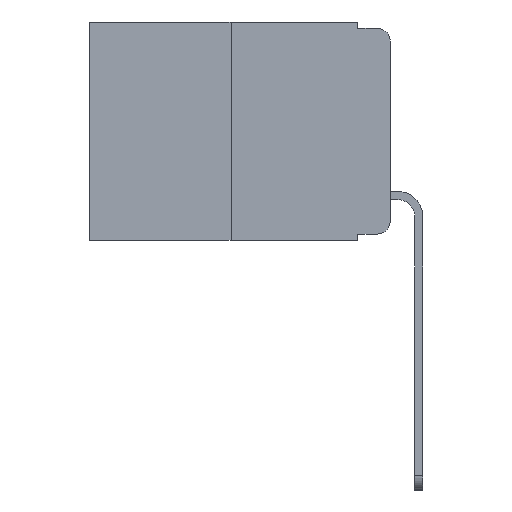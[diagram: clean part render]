
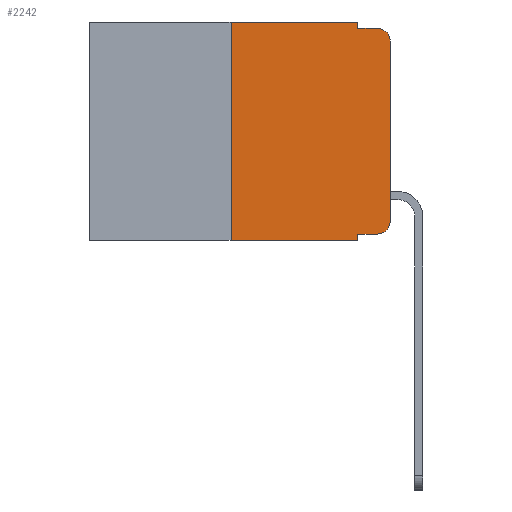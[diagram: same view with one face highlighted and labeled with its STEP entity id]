
A CAD part, left-side view. The second image highlights one B-rep face of the part: STEP entity #2242.
In plain terms, the highlighted planar face has unit normal (-1, 0, 0).
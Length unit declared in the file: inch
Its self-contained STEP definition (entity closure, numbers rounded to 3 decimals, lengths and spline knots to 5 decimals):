
#78 = CARTESIAN_POINT ( 'NONE',  ( 0., 0.02, -0.333 ) ) ;
#132 = ORIENTED_EDGE ( 'NONE', *, *, #5493, .T. ) ;
#472 = CARTESIAN_POINT ( 'NONE',  ( 0., 0.051, -0.333 ) ) ;
#522 = ORIENTED_EDGE ( 'NONE', *, *, #5585, .T. ) ;
#524 = CARTESIAN_POINT ( 'NONE',  ( 0., 0.02, -0.313 ) ) ;
#1256 = VECTOR ( 'NONE', #2995, 39.37008 ) ;
#1298 = ORIENTED_EDGE ( 'NONE', *, *, #5512, .F. ) ;
#1524 = EDGE_LOOP ( 'NONE', ( #5751, #132, #1298, #4695, #6941, #10758, #8282, #1946, #522, #3207 ) ) ;
#1672 = LINE ( 'NONE', #10597, #6989 ) ;
#1694 = VERTEX_POINT ( 'NONE', #8620 ) ;
#1697 = DIRECTION ( 'NONE',  ( 0., -1., 0. ) ) ;
#1806 = DIRECTION ( 'NONE',  ( 0., 0., -1. ) ) ;
#1946 = ORIENTED_EDGE ( 'NONE', *, *, #5566, .F. ) ;
#2242 = ADVANCED_FACE ( 'NONE', ( #3679 ), #8154, .F. ) ;
#2278 = VECTOR ( 'NONE', #11358, 39.37008 ) ;
#2470 = CARTESIAN_POINT ( 'NONE',  ( 0., 0., -0.313 ) ) ;
#2820 = VECTOR ( 'NONE', #9596, 39.37008 ) ;
#2995 = DIRECTION ( 'NONE',  ( 0., 0., -1. ) ) ;
#3207 = ORIENTED_EDGE ( 'NONE', *, *, #5589, .T. ) ;
#3339 = VECTOR ( 'NONE', #6860, 39.37008 ) ;
#3516 = VERTEX_POINT ( 'NONE', #12170 ) ;
#3679 = FACE_OUTER_BOUND ( 'NONE', #1524, .T. ) ;
#3971 = CARTESIAN_POINT ( 'NONE',  ( 0., 0.051, -0.343 ) ) ;
#3986 = CARTESIAN_POINT ( 'NONE',  ( 0., 0.02, -0.03 ) ) ;
#4695 = ORIENTED_EDGE ( 'NONE', *, *, #5534, .F. ) ;
#4954 = EDGE_CURVE ( 'NONE', #11299, #1694, #8013, .T. ) ;
#5103 = DIRECTION ( 'NONE',  ( 0., 0., -1. ) ) ;
#5192 = DIRECTION ( 'NONE',  ( 0., -1., 0. ) ) ;
#5389 = LINE ( 'NONE', #7901, #9918 ) ;
#5473 = EDGE_CURVE ( 'NONE', #10146, #3516, #10505, .T. ) ;
#5493 = EDGE_CURVE ( 'NONE', #3516, #11054, #10216, .T. ) ;
#5512 = EDGE_CURVE ( 'NONE', #8176, #11054, #5389, .T. ) ;
#5534 = EDGE_CURVE ( 'NONE', #1694, #8176, #12015, .T. ) ;
#5545 = EDGE_CURVE ( 'NONE', #9021, #11299, #1672, .T. ) ;
#5566 = EDGE_CURVE ( 'NONE', #5857, #8592, #7274, .T. ) ;
#5585 = EDGE_CURVE ( 'NONE', #5857, #6672, #9077, .T. ) ;
#5589 = EDGE_CURVE ( 'NONE', #6672, #10146, #11449, .T. ) ;
#5729 = CARTESIAN_POINT ( 'NONE',  ( 0., 0.051, -0.01 ) ) ;
#5751 = ORIENTED_EDGE ( 'NONE', *, *, #5473, .T. ) ;
#5857 = VERTEX_POINT ( 'NONE', #8258 ) ;
#5927 = CARTESIAN_POINT ( 'NONE',  ( 0., 0.473, -0.343 ) ) ;
#6172 = EDGE_CURVE ( 'NONE', #9021, #8592, #10883, .T. ) ;
#6672 = VERTEX_POINT ( 'NONE', #78 ) ;
#6710 = VECTOR ( 'NONE', #5192, 39.37008 ) ;
#6860 = DIRECTION ( 'NONE',  ( 0., -1., 0. ) ) ;
#6941 = ORIENTED_EDGE ( 'NONE', *, *, #4954, .F. ) ;
#6989 = VECTOR ( 'NONE', #12360, 39.37008 ) ;
#7274 = LINE ( 'NONE', #8813, #1256 ) ;
#7455 = AXIS2_PLACEMENT_3D ( 'NONE', #8609, #9931, #11665 ) ;
#7819 = CARTESIAN_POINT ( 'NONE',  ( 0., 0., 0. ) ) ;
#7828 = CARTESIAN_POINT ( 'NONE',  ( 0., 0.473, 0. ) ) ;
#7901 = CARTESIAN_POINT ( 'NONE',  ( 0., 0.051, -0.01 ) ) ;
#7981 = DIRECTION ( 'NONE',  ( -1., 0., 0. ) ) ;
#8013 = LINE ( 'NONE', #7828, #2278 ) ;
#8154 = PLANE ( 'NONE',  #7455 ) ;
#8176 = VERTEX_POINT ( 'NONE', #5729 ) ;
#8258 = CARTESIAN_POINT ( 'NONE',  ( 0., 0.051, -0.333 ) ) ;
#8282 = ORIENTED_EDGE ( 'NONE', *, *, #6172, .T. ) ;
#8592 = VERTEX_POINT ( 'NONE', #3971 ) ;
#8609 = CARTESIAN_POINT ( 'NONE',  ( 0., 0.473, 0. ) ) ;
#8620 = CARTESIAN_POINT ( 'NONE',  ( 0., 0.051, 0. ) ) ;
#8774 = CARTESIAN_POINT ( 'NONE',  ( 0., 0.051, 0. ) ) ;
#8813 = CARTESIAN_POINT ( 'NONE',  ( 0., 0.051, 0. ) ) ;
#9021 = VERTEX_POINT ( 'NONE', #9598 ) ;
#9077 = LINE ( 'NONE', #472, #6710 ) ;
#9596 = DIRECTION ( 'NONE',  ( 0., 0., 1. ) ) ;
#9598 = CARTESIAN_POINT ( 'NONE',  ( 0., 0.25, -0.343 ) ) ;
#9918 = VECTOR ( 'NONE', #1697, 39.37008 ) ;
#9931 = DIRECTION ( 'NONE',  ( 1., 0., 0. ) ) ;
#10017 = CARTESIAN_POINT ( 'NONE',  ( 0., 0.25, 0. ) ) ;
#10146 = VERTEX_POINT ( 'NONE', #2470 ) ;
#10216 = CIRCLE ( 'NONE', #11492, 0.02 ) ;
#10505 = LINE ( 'NONE', #7819, #2820 ) ;
#10557 = DIRECTION ( 'NONE',  ( -1., 0., 0. ) ) ;
#10597 = CARTESIAN_POINT ( 'NONE',  ( 0., 0.25, 0. ) ) ;
#10758 = ORIENTED_EDGE ( 'NONE', *, *, #5545, .F. ) ;
#10883 = LINE ( 'NONE', #5927, #3339 ) ;
#11054 = VERTEX_POINT ( 'NONE', #12497 ) ;
#11299 = VERTEX_POINT ( 'NONE', #10017 ) ;
#11358 = DIRECTION ( 'NONE',  ( 0., -1., 0. ) ) ;
#11441 = AXIS2_PLACEMENT_3D ( 'NONE', #524, #7981, #1806 ) ;
#11449 = CIRCLE ( 'NONE', #11441, 0.02 ) ;
#11492 = AXIS2_PLACEMENT_3D ( 'NONE', #3986, #10557, #5103 ) ;
#11665 = DIRECTION ( 'NONE',  ( 0., 0., -1. ) ) ;
#11731 = VECTOR ( 'NONE', #12323, 39.37008 ) ;
#12015 = LINE ( 'NONE', #8774, #11731 ) ;
#12170 = CARTESIAN_POINT ( 'NONE',  ( 0., 0., -0.03 ) ) ;
#12323 = DIRECTION ( 'NONE',  ( 0., 0., -1. ) ) ;
#12360 = DIRECTION ( 'NONE',  ( 0., 0., 1. ) ) ;
#12497 = CARTESIAN_POINT ( 'NONE',  ( 0., 0.02, -0.01 ) ) ;
